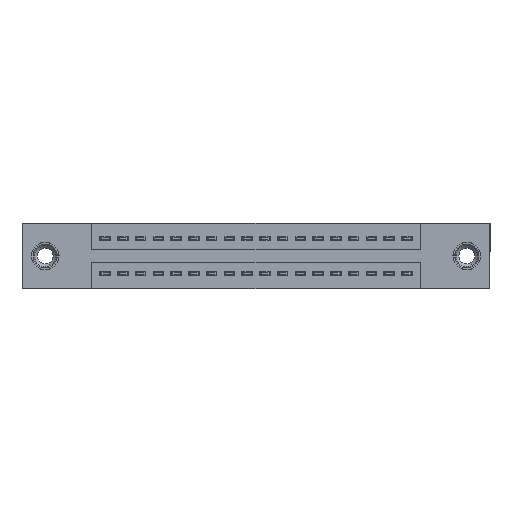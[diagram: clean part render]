
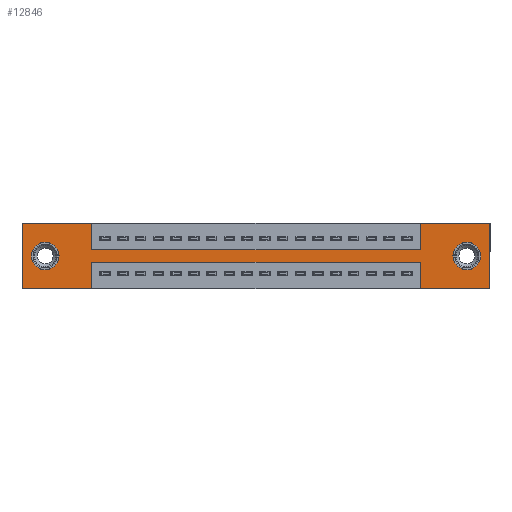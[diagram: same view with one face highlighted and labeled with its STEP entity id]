
A CAD part, front view. The second image highlights one B-rep face of the part: STEP entity #12846.
In plain terms, the highlighted planar face has unit normal (0, -1, 0).
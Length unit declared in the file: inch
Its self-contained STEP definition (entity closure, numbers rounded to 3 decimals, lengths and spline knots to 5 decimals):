
#258 = CARTESIAN_POINT ( 'NONE',  ( 2.2425, 0., -0.37 ) ) ;
#344 = DIRECTION ( 'NONE',  ( -1., 0., 0. ) ) ;
#363 = CARTESIAN_POINT ( 'NONE',  ( 2.2425, 0., -0.15 ) ) ;
#570 = CARTESIAN_POINT ( 'NONE',  ( 0.3925, 0., -0.15 ) ) ;
#641 = DIRECTION ( 'NONE',  ( 0., 0., -1. ) ) ;
#813 = LINE ( 'NONE', #13178, #12316 ) ;
#1043 = EDGE_CURVE ( 'NONE', #17447, #3816, #7511, .T. ) ;
#1061 = EDGE_CURVE ( 'NONE', #15175, #10851, #3980, .T. ) ;
#1067 = VERTEX_POINT ( 'NONE', #9801 ) ;
#1093 = LINE ( 'NONE', #4630, #4686 ) ;
#1177 = CARTESIAN_POINT ( 'NONE',  ( 0., 0., -0.37 ) ) ;
#1202 = EDGE_CURVE ( 'NONE', #15565, #11937, #1093, .T. ) ;
#1238 = VECTOR ( 'NONE', #3591, 39.37008 ) ;
#1281 = EDGE_LOOP ( 'NONE', ( #17156, #16293 ) ) ;
#1356 = ORIENTED_EDGE ( 'NONE', *, *, #1043, .T. ) ;
#1630 = CARTESIAN_POINT ( 'NONE',  ( 0.3925, 0., -0.22 ) ) ;
#1645 = EDGE_CURVE ( 'NONE', #14443, #4570, #3613, .T. ) ;
#1657 = ORIENTED_EDGE ( 'NONE', *, *, #2040, .F. ) ;
#1698 = EDGE_CURVE ( 'NONE', #3816, #17447, #14588, .T. ) ;
#1726 = ORIENTED_EDGE ( 'NONE', *, *, #11378, .F. ) ;
#2026 = ORIENTED_EDGE ( 'NONE', *, *, #1061, .F. ) ;
#2040 = EDGE_CURVE ( 'NONE', #17799, #6134, #5516, .T. ) ;
#2195 = EDGE_CURVE ( 'NONE', #12629, #5969, #18449, .T. ) ;
#2617 = DIRECTION ( 'NONE',  ( 1., 0., 0. ) ) ;
#2633 = VECTOR ( 'NONE', #2617, 39.37008 ) ;
#3044 = CARTESIAN_POINT ( 'NONE',  ( 2.505, 0., -0.263 ) ) ;
#3171 = CARTESIAN_POINT ( 'NONE',  ( 2.505, 0., -0.107 ) ) ;
#3488 = EDGE_CURVE ( 'NONE', #4570, #18862, #5465, .T. ) ;
#3591 = DIRECTION ( 'NONE',  ( 0., 0., -1. ) ) ;
#3613 = LINE ( 'NONE', #6470, #18929 ) ;
#3660 = ORIENTED_EDGE ( 'NONE', *, *, #1698, .T. ) ;
#3661 = DIRECTION ( 'NONE',  ( 0., 0., 1. ) ) ;
#3710 = DIRECTION ( 'NONE',  ( 1., 0., 0. ) ) ;
#3761 = ORIENTED_EDGE ( 'NONE', *, *, #1645, .F. ) ;
#3816 = VERTEX_POINT ( 'NONE', #15247 ) ;
#3920 = ORIENTED_EDGE ( 'NONE', *, *, #18206, .F. ) ;
#3980 = LINE ( 'NONE', #17254, #7053 ) ;
#4040 = AXIS2_PLACEMENT_3D ( 'NONE', #12970, #4043, #14463 ) ;
#4043 = DIRECTION ( 'NONE',  ( 0., 1., 0. ) ) ;
#4234 = DIRECTION ( 'NONE',  ( 0., 1., 0. ) ) ;
#4334 = VECTOR ( 'NONE', #344, 39.37008 ) ;
#4570 = VERTEX_POINT ( 'NONE', #15488 ) ;
#4620 = DIRECTION ( 'NONE',  ( 1., 0., 0. ) ) ;
#4630 = CARTESIAN_POINT ( 'NONE',  ( 0.3925, 0., -0.37 ) ) ;
#4686 = VECTOR ( 'NONE', #4783, 39.37008 ) ;
#4783 = DIRECTION ( 'NONE',  ( 0., 0., -1. ) ) ;
#4815 = LINE ( 'NONE', #10818, #4334 ) ;
#5318 = LINE ( 'NONE', #11026, #1238 ) ;
#5465 = LINE ( 'NONE', #11679, #15890 ) ;
#5516 = LINE ( 'NONE', #14142, #17319 ) ;
#5635 = CARTESIAN_POINT ( 'NONE',  ( 0., 0., 0. ) ) ;
#5740 = CARTESIAN_POINT ( 'NONE',  ( 0.13, 0., -0.185 ) ) ;
#5793 = DIRECTION ( 'NONE',  ( -1., 0., 0. ) ) ;
#5867 = CARTESIAN_POINT ( 'NONE',  ( 0.13, 0., -0.263 ) ) ;
#5969 = VERTEX_POINT ( 'NONE', #3044 ) ;
#5994 = ORIENTED_EDGE ( 'NONE', *, *, #10875, .F. ) ;
#6134 = VERTEX_POINT ( 'NONE', #363 ) ;
#6384 = ORIENTED_EDGE ( 'NONE', *, *, #8630, .F. ) ;
#6442 = CARTESIAN_POINT ( 'NONE',  ( 2.2425, 0., 0. ) ) ;
#6470 = CARTESIAN_POINT ( 'NONE',  ( 2.635, 0., 0. ) ) ;
#6481 = EDGE_CURVE ( 'NONE', #18862, #8708, #813, .T. ) ;
#6554 = AXIS2_PLACEMENT_3D ( 'NONE', #10858, #16680, #10910 ) ;
#7053 = VECTOR ( 'NONE', #17208, 39.37008 ) ;
#7349 = EDGE_LOOP ( 'NONE', ( #15696, #3920, #7570, #10183, #3761, #6384, #8967, #1657, #5994, #7460, #2026, #1726 ) ) ;
#7460 = ORIENTED_EDGE ( 'NONE', *, *, #11693, .F. ) ;
#7462 = CARTESIAN_POINT ( 'NONE',  ( 2.505, 0., -0.185 ) ) ;
#7511 = CIRCLE ( 'NONE', #6554, 0.078 ) ;
#7570 = ORIENTED_EDGE ( 'NONE', *, *, #6481, .F. ) ;
#7730 = LINE ( 'NONE', #13535, #18582 ) ;
#7922 = DIRECTION ( 'NONE',  ( 0., 0., 1. ) ) ;
#8630 = EDGE_CURVE ( 'NONE', #17100, #14443, #7730, .T. ) ;
#8708 = VERTEX_POINT ( 'NONE', #18135 ) ;
#8910 = DIRECTION ( 'NONE',  ( 0., 0., -1. ) ) ;
#8967 = ORIENTED_EDGE ( 'NONE', *, *, #14940, .F. ) ;
#9669 = DIRECTION ( 'NONE',  ( 0., -1., 0. ) ) ;
#9801 = CARTESIAN_POINT ( 'NONE',  ( 0.3925, 0., 0. ) ) ;
#10183 = ORIENTED_EDGE ( 'NONE', *, *, #3488, .F. ) ;
#10252 = VECTOR ( 'NONE', #7922, 39.37008 ) ;
#10457 = EDGE_CURVE ( 'NONE', #5969, #12629, #16677, .T. ) ;
#10606 = VECTOR ( 'NONE', #16515, 39.37008 ) ;
#10818 = CARTESIAN_POINT ( 'NONE',  ( 0., 0., -0.37 ) ) ;
#10851 = VERTEX_POINT ( 'NONE', #12456 ) ;
#10858 = CARTESIAN_POINT ( 'NONE',  ( 0.13, 0., -0.185 ) ) ;
#10875 = EDGE_CURVE ( 'NONE', #1067, #17799, #5318, .T. ) ;
#10910 = DIRECTION ( 'NONE',  ( 0., 0., 1. ) ) ;
#11026 = CARTESIAN_POINT ( 'NONE',  ( 0.3925, 0., 0. ) ) ;
#11068 = FACE_OUTER_BOUND ( 'NONE', #7349, .T. ) ;
#11072 = LINE ( 'NONE', #1630, #10606 ) ;
#11378 = EDGE_CURVE ( 'NONE', #11937, #15175, #4815, .T. ) ;
#11679 = CARTESIAN_POINT ( 'NONE',  ( 0., 0., -0.37 ) ) ;
#11693 = EDGE_CURVE ( 'NONE', #10851, #1067, #18457, .T. ) ;
#11937 = VERTEX_POINT ( 'NONE', #18017 ) ;
#12316 = VECTOR ( 'NONE', #14668, 39.37008 ) ;
#12456 = CARTESIAN_POINT ( 'NONE',  ( 0., 0., 0. ) ) ;
#12594 = CARTESIAN_POINT ( 'NONE',  ( 0., 0., -0.37 ) ) ;
#12629 = VERTEX_POINT ( 'NONE', #3171 ) ;
#12846 = ADVANCED_FACE ( 'NONE', ( #18440, #18901, #11068 ), #18512, .T. ) ;
#12970 = CARTESIAN_POINT ( 'NONE',  ( 2.505, 0., -0.185 ) ) ;
#13018 = EDGE_LOOP ( 'NONE', ( #3660, #1356 ) ) ;
#13178 = CARTESIAN_POINT ( 'NONE',  ( 2.2425, 0., -0.37 ) ) ;
#13535 = CARTESIAN_POINT ( 'NONE',  ( 0., 0., 0. ) ) ;
#13954 = CARTESIAN_POINT ( 'NONE',  ( 0.3925, 0., -0.22 ) ) ;
#14142 = CARTESIAN_POINT ( 'NONE',  ( 0.3925, 0., -0.15 ) ) ;
#14204 = LINE ( 'NONE', #6442, #10252 ) ;
#14443 = VERTEX_POINT ( 'NONE', #17125 ) ;
#14463 = DIRECTION ( 'NONE',  ( 0., 0., -1. ) ) ;
#14588 = CIRCLE ( 'NONE', #17701, 0.078 ) ;
#14668 = DIRECTION ( 'NONE',  ( 0., 0., 1. ) ) ;
#14940 = EDGE_CURVE ( 'NONE', #6134, #17100, #14204, .T. ) ;
#15175 = VERTEX_POINT ( 'NONE', #1177 ) ;
#15247 = CARTESIAN_POINT ( 'NONE',  ( 0.13, 0., -0.107 ) ) ;
#15485 = CARTESIAN_POINT ( 'NONE',  ( 2.2425, 0., 0. ) ) ;
#15488 = CARTESIAN_POINT ( 'NONE',  ( 2.635, 0., -0.37 ) ) ;
#15565 = VERTEX_POINT ( 'NONE', #13954 ) ;
#15696 = ORIENTED_EDGE ( 'NONE', *, *, #1202, .F. ) ;
#15890 = VECTOR ( 'NONE', #5793, 39.37008 ) ;
#16293 = ORIENTED_EDGE ( 'NONE', *, *, #10457, .T. ) ;
#16515 = DIRECTION ( 'NONE',  ( -1., 0., 0. ) ) ;
#16677 = CIRCLE ( 'NONE', #18199, 0.078 ) ;
#16680 = DIRECTION ( 'NONE',  ( 0., 1., 0. ) ) ;
#17100 = VERTEX_POINT ( 'NONE', #15485 ) ;
#17125 = CARTESIAN_POINT ( 'NONE',  ( 2.635, 0., 0. ) ) ;
#17156 = ORIENTED_EDGE ( 'NONE', *, *, #2195, .T. ) ;
#17208 = DIRECTION ( 'NONE',  ( 0., 0., 1. ) ) ;
#17254 = CARTESIAN_POINT ( 'NONE',  ( 0., 0., 0. ) ) ;
#17319 = VECTOR ( 'NONE', #3710, 39.37008 ) ;
#17447 = VERTEX_POINT ( 'NONE', #5867 ) ;
#17630 = AXIS2_PLACEMENT_3D ( 'NONE', #12594, #9669, #641 ) ;
#17701 = AXIS2_PLACEMENT_3D ( 'NONE', #5740, #4234, #3661 ) ;
#17770 = DIRECTION ( 'NONE',  ( 0., 1., 0. ) ) ;
#17799 = VERTEX_POINT ( 'NONE', #570 ) ;
#18017 = CARTESIAN_POINT ( 'NONE',  ( 0.3925, 0., -0.37 ) ) ;
#18135 = CARTESIAN_POINT ( 'NONE',  ( 2.2425, 0., -0.22 ) ) ;
#18199 = AXIS2_PLACEMENT_3D ( 'NONE', #7462, #17770, #8910 ) ;
#18206 = EDGE_CURVE ( 'NONE', #8708, #15565, #11072, .T. ) ;
#18440 = FACE_BOUND ( 'NONE', #1281, .T. ) ;
#18449 = CIRCLE ( 'NONE', #4040, 0.078 ) ;
#18457 = LINE ( 'NONE', #5635, #2633 ) ;
#18512 = PLANE ( 'NONE',  #17630 ) ;
#18582 = VECTOR ( 'NONE', #4620, 39.37008 ) ;
#18846 = DIRECTION ( 'NONE',  ( 0., 0., -1. ) ) ;
#18862 = VERTEX_POINT ( 'NONE', #258 ) ;
#18901 = FACE_BOUND ( 'NONE', #13018, .T. ) ;
#18929 = VECTOR ( 'NONE', #18846, 39.37008 ) ;
